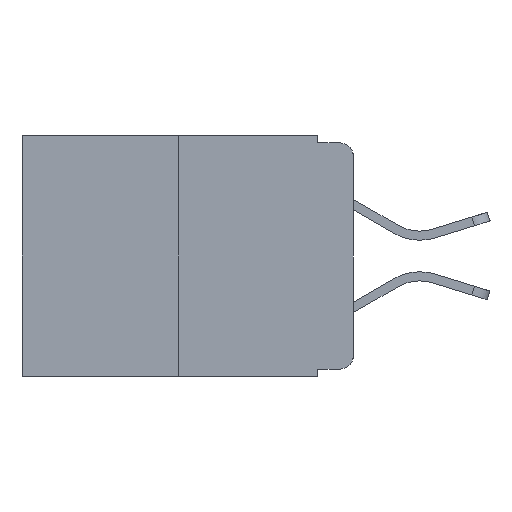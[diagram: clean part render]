
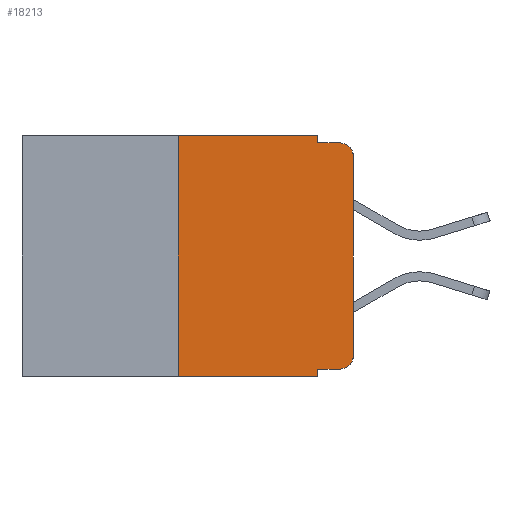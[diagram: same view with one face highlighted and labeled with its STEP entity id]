
A CAD part, left-side view. The second image highlights one B-rep face of the part: STEP entity #18213.
In plain terms, the highlighted planar face has unit normal (-1, 0, 0).
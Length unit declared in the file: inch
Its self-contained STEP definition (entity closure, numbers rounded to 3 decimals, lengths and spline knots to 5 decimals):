
#245 = LINE ( 'NONE', #16106, #12159 ) ;
#411 = CARTESIAN_POINT ( 'NONE',  ( 0., 0.051, -0.333 ) ) ;
#1156 = FACE_OUTER_BOUND ( 'NONE', #10814, .T. ) ;
#1229 = AXIS2_PLACEMENT_3D ( 'NONE', #15241, #10978, #5138 ) ;
#1574 = EDGE_CURVE ( 'NONE', #6495, #18067, #2230, .T. ) ;
#1975 = VECTOR ( 'NONE', #14703, 39.37008 ) ;
#2035 = VECTOR ( 'NONE', #5351, 39.37008 ) ;
#2064 = ORIENTED_EDGE ( 'NONE', *, *, #2356, .F. ) ;
#2139 = DIRECTION ( 'NONE',  ( 0., 0., -1. ) ) ;
#2230 = LINE ( 'NONE', #7884, #11163 ) ;
#2316 = DIRECTION ( 'NONE',  ( -1., 0., 0. ) ) ;
#2356 = EDGE_CURVE ( 'NONE', #6495, #5633, #10626, .T. ) ;
#2745 = DIRECTION ( 'NONE',  ( 0., -1., 0. ) ) ;
#3716 = DIRECTION ( 'NONE',  ( 0., -1., 0. ) ) ;
#3795 = CARTESIAN_POINT ( 'NONE',  ( 0., 0.051, -0.01 ) ) ;
#3966 = LINE ( 'NONE', #9617, #6659 ) ;
#4672 = VECTOR ( 'NONE', #2745, 39.37008 ) ;
#4869 = CARTESIAN_POINT ( 'NONE',  ( 0., 0.02, -0.333 ) ) ;
#4891 = CARTESIAN_POINT ( 'NONE',  ( 0., 0., 0. ) ) ;
#4954 = ORIENTED_EDGE ( 'NONE', *, *, #14389, .T. ) ;
#5032 = CARTESIAN_POINT ( 'NONE',  ( 0., 0.02, -0.01 ) ) ;
#5115 = VERTEX_POINT ( 'NONE', #15964 ) ;
#5138 = DIRECTION ( 'NONE',  ( 0., 0., -1. ) ) ;
#5315 = PLANE ( 'NONE',  #1229 ) ;
#5351 = DIRECTION ( 'NONE',  ( 0., -1., 0. ) ) ;
#5488 = VERTEX_POINT ( 'NONE', #11843 ) ;
#5633 = VERTEX_POINT ( 'NONE', #17970 ) ;
#5741 = EDGE_CURVE ( 'NONE', #12604, #17455, #3966, .T. ) ;
#5986 = ORIENTED_EDGE ( 'NONE', *, *, #17103, .T. ) ;
#5999 = LINE ( 'NONE', #4891, #12164 ) ;
#6495 = VERTEX_POINT ( 'NONE', #411 ) ;
#6643 = EDGE_CURVE ( 'NONE', #5488, #5115, #7915, .T. ) ;
#6659 = VECTOR ( 'NONE', #15363, 39.37008 ) ;
#7045 = ORIENTED_EDGE ( 'NONE', *, *, #12929, .T. ) ;
#7116 = CARTESIAN_POINT ( 'NONE',  ( 0., 0.25, 0. ) ) ;
#7238 = VERTEX_POINT ( 'NONE', #8420 ) ;
#7671 = EDGE_CURVE ( 'NONE', #12604, #5633, #11165, .T. ) ;
#7878 = DIRECTION ( 'NONE',  ( -1., 0., 0. ) ) ;
#7884 = CARTESIAN_POINT ( 'NONE',  ( 0., 0.051, -0.333 ) ) ;
#7915 = LINE ( 'NONE', #13569, #14695 ) ;
#7984 = VERTEX_POINT ( 'NONE', #10516 ) ;
#8420 = CARTESIAN_POINT ( 'NONE',  ( 0., 0., -0.03 ) ) ;
#8680 = DIRECTION ( 'NONE',  ( 0., -1., 0. ) ) ;
#9088 = CARTESIAN_POINT ( 'NONE',  ( 0., 0.02, -0.313 ) ) ;
#9101 = VERTEX_POINT ( 'NONE', #5032 ) ;
#9314 = CIRCLE ( 'NONE', #13479, 0.02 ) ;
#9617 = CARTESIAN_POINT ( 'NONE',  ( 0., 0.25, 0. ) ) ;
#9726 = CARTESIAN_POINT ( 'NONE',  ( 0., 0.25, -0.343 ) ) ;
#9808 = ORIENTED_EDGE ( 'NONE', *, *, #17887, .F. ) ;
#10092 = EDGE_CURVE ( 'NONE', #5115, #9101, #18064, .T. ) ;
#10452 = AXIS2_PLACEMENT_3D ( 'NONE', #9088, #2316, #2139 ) ;
#10516 = CARTESIAN_POINT ( 'NONE',  ( 0., 0., -0.313 ) ) ;
#10542 = ORIENTED_EDGE ( 'NONE', *, *, #6643, .F. ) ;
#10626 = LINE ( 'NONE', #13130, #1975 ) ;
#10814 = EDGE_LOOP ( 'NONE', ( #7045, #5986, #13931, #10542, #9808, #12187, #16652, #2064, #17004, #4954 ) ) ;
#10844 = CARTESIAN_POINT ( 'NONE',  ( 0., 0.02, -0.03 ) ) ;
#10978 = DIRECTION ( 'NONE',  ( 1., 0., 0. ) ) ;
#11034 = CIRCLE ( 'NONE', #10452, 0.02 ) ;
#11163 = VECTOR ( 'NONE', #3716, 39.37008 ) ;
#11165 = LINE ( 'NONE', #16839, #4672 ) ;
#11843 = CARTESIAN_POINT ( 'NONE',  ( 0., 0.051, 0. ) ) ;
#12159 = VECTOR ( 'NONE', #8680, 39.37008 ) ;
#12164 = VECTOR ( 'NONE', #17606, 39.37008 ) ;
#12187 = ORIENTED_EDGE ( 'NONE', *, *, #5741, .F. ) ;
#12604 = VERTEX_POINT ( 'NONE', #9726 ) ;
#12929 = EDGE_CURVE ( 'NONE', #7984, #7238, #5999, .T. ) ;
#13130 = CARTESIAN_POINT ( 'NONE',  ( 0., 0.051, 0. ) ) ;
#13479 = AXIS2_PLACEMENT_3D ( 'NONE', #10844, #7878, #13627 ) ;
#13569 = CARTESIAN_POINT ( 'NONE',  ( 0., 0.051, 0. ) ) ;
#13627 = DIRECTION ( 'NONE',  ( 0., 0., -1. ) ) ;
#13655 = DIRECTION ( 'NONE',  ( 0., 0., -1. ) ) ;
#13931 = ORIENTED_EDGE ( 'NONE', *, *, #10092, .F. ) ;
#14389 = EDGE_CURVE ( 'NONE', #18067, #7984, #11034, .T. ) ;
#14695 = VECTOR ( 'NONE', #13655, 39.37008 ) ;
#14703 = DIRECTION ( 'NONE',  ( 0., 0., -1. ) ) ;
#15241 = CARTESIAN_POINT ( 'NONE',  ( 0., 0.473, 0. ) ) ;
#15363 = DIRECTION ( 'NONE',  ( 0., 0., 1. ) ) ;
#15964 = CARTESIAN_POINT ( 'NONE',  ( 0., 0.051, -0.01 ) ) ;
#16106 = CARTESIAN_POINT ( 'NONE',  ( 0., 0.473, 0. ) ) ;
#16652 = ORIENTED_EDGE ( 'NONE', *, *, #7671, .T. ) ;
#16839 = CARTESIAN_POINT ( 'NONE',  ( 0., 0.473, -0.343 ) ) ;
#17004 = ORIENTED_EDGE ( 'NONE', *, *, #1574, .T. ) ;
#17103 = EDGE_CURVE ( 'NONE', #7238, #9101, #9314, .T. ) ;
#17455 = VERTEX_POINT ( 'NONE', #7116 ) ;
#17606 = DIRECTION ( 'NONE',  ( 0., 0., 1. ) ) ;
#17887 = EDGE_CURVE ( 'NONE', #17455, #5488, #245, .T. ) ;
#17970 = CARTESIAN_POINT ( 'NONE',  ( 0., 0.051, -0.343 ) ) ;
#18064 = LINE ( 'NONE', #3795, #2035 ) ;
#18067 = VERTEX_POINT ( 'NONE', #4869 ) ;
#18213 = ADVANCED_FACE ( 'NONE', ( #1156 ), #5315, .F. ) ;
